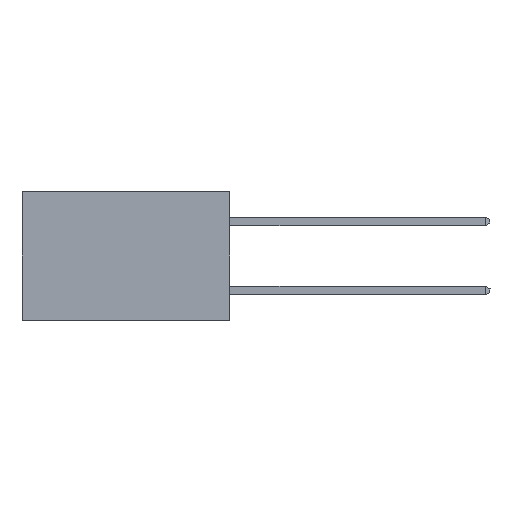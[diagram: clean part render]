
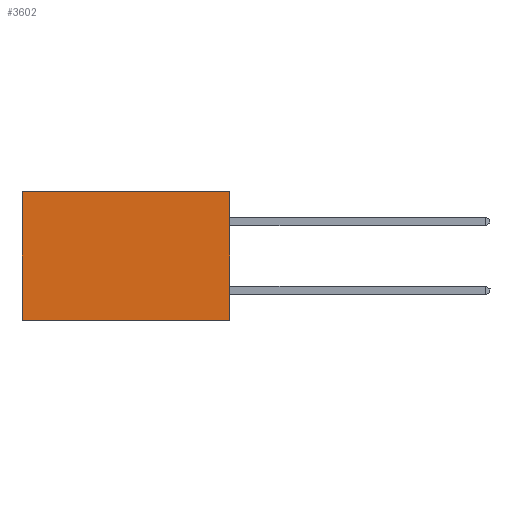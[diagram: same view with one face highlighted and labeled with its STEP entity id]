
A CAD part, left-side view. The second image highlights one B-rep face of the part: STEP entity #3602.
In plain terms, the highlighted planar face has unit normal (-1, 0, 0).
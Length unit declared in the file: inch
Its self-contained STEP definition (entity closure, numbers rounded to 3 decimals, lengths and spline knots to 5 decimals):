
#74 = PLANE ( 'NONE',  #5545 ) ;
#957 = VECTOR ( 'NONE', #24305, 39.37008 ) ;
#1686 = CARTESIAN_POINT ( 'NONE',  ( 0.298, 0., 0. ) ) ;
#1715 = LINE ( 'NONE', #6351, #957 ) ;
#3150 = DIRECTION ( 'NONE',  ( 1., 0., 0. ) ) ;
#3602 = ADVANCED_FACE ( 'NONE', ( #4133 ), #74, .F. ) ;
#3704 = VECTOR ( 'NONE', #15773, 39.37008 ) ;
#4068 = EDGE_CURVE ( 'NONE', #8117, #28165, #28543, .T. ) ;
#4133 = FACE_OUTER_BOUND ( 'NONE', #22888, .T. ) ;
#4264 = EDGE_CURVE ( 'NONE', #28165, #25979, #1715, .T. ) ;
#5029 = LINE ( 'NONE', #14440, #15876 ) ;
#5545 = AXIS2_PLACEMENT_3D ( 'NONE', #24604, #3150, #22643 ) ;
#5676 = VERTEX_POINT ( 'NONE', #5903 ) ;
#5903 = CARTESIAN_POINT ( 'NONE',  ( 0.298, 0.6, 0. ) ) ;
#6329 = CARTESIAN_POINT ( 'NONE',  ( 0.298, 0., -0.37 ) ) ;
#6351 = CARTESIAN_POINT ( 'NONE',  ( 0.298, 0., -0.37 ) ) ;
#8117 = VERTEX_POINT ( 'NONE', #1686 ) ;
#11209 = LINE ( 'NONE', #31297, #31282 ) ;
#14440 = CARTESIAN_POINT ( 'NONE',  ( 0.298, 0., 0. ) ) ;
#14498 = ORIENTED_EDGE ( 'NONE', *, *, #4068, .F. ) ;
#15773 = DIRECTION ( 'NONE',  ( 0., 0., -1. ) ) ;
#15876 = VECTOR ( 'NONE', #16929, 39.37008 ) ;
#16929 = DIRECTION ( 'NONE',  ( 0., 1., 0. ) ) ;
#18228 = EDGE_CURVE ( 'NONE', #8117, #5676, #5029, .T. ) ;
#19883 = CARTESIAN_POINT ( 'NONE',  ( 0.298, 0.6, -0.37 ) ) ;
#21968 = ORIENTED_EDGE ( 'NONE', *, *, #18228, .T. ) ;
#22643 = DIRECTION ( 'NONE',  ( 0., 0., -1. ) ) ;
#22888 = EDGE_LOOP ( 'NONE', ( #25024, #30708, #14498, #21968 ) ) ;
#24305 = DIRECTION ( 'NONE',  ( 0., 1., 0. ) ) ;
#24604 = CARTESIAN_POINT ( 'NONE',  ( 0.298, 0., 0. ) ) ;
#24774 = DIRECTION ( 'NONE',  ( 0., 0., -1. ) ) ;
#25024 = ORIENTED_EDGE ( 'NONE', *, *, #29895, .T. ) ;
#25979 = VERTEX_POINT ( 'NONE', #19883 ) ;
#28152 = CARTESIAN_POINT ( 'NONE',  ( 0.298, 0., 0. ) ) ;
#28165 = VERTEX_POINT ( 'NONE', #6329 ) ;
#28543 = LINE ( 'NONE', #28152, #3704 ) ;
#29895 = EDGE_CURVE ( 'NONE', #5676, #25979, #11209, .T. ) ;
#30708 = ORIENTED_EDGE ( 'NONE', *, *, #4264, .F. ) ;
#31282 = VECTOR ( 'NONE', #24774, 39.37008 ) ;
#31297 = CARTESIAN_POINT ( 'NONE',  ( 0.298, 0.6, 0. ) ) ;
